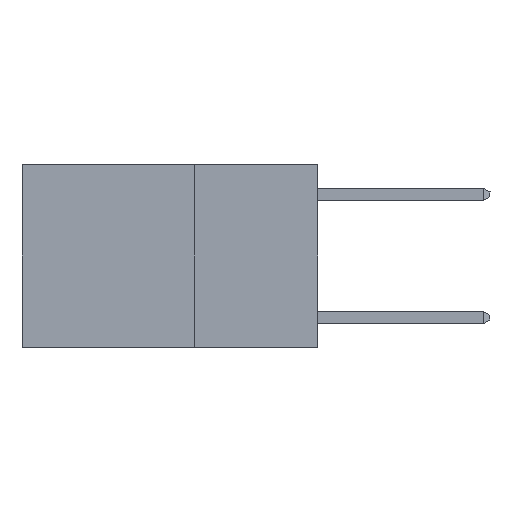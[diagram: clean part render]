
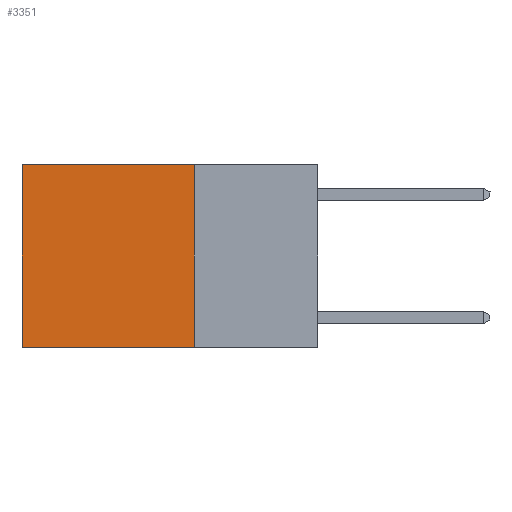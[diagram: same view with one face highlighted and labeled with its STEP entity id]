
A CAD part, left-side view. The second image highlights one B-rep face of the part: STEP entity #3351.
In plain terms, the highlighted planar face has unit normal (-1, 0, 0).
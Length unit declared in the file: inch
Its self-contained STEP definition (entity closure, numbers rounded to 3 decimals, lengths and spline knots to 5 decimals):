
#272 = VECTOR ( 'NONE', #531, 39.37008 ) ;
#531 = DIRECTION ( 'NONE',  ( 0., 0., -1. ) ) ;
#1153 = VERTEX_POINT ( 'NONE', #8296 ) ;
#1185 = CARTESIAN_POINT ( 'NONE',  ( 0.2625, 0.6, -0.37 ) ) ;
#1396 = LINE ( 'NONE', #9243, #9257 ) ;
#1548 = LINE ( 'NONE', #5243, #272 ) ;
#2403 = VERTEX_POINT ( 'NONE', #1185 ) ;
#2788 = VERTEX_POINT ( 'NONE', #6222 ) ;
#3244 = EDGE_LOOP ( 'NONE', ( #3820, #5809, #5583, #9516 ) ) ;
#3351 = ADVANCED_FACE ( 'NONE', ( #9793 ), #3911, .F. ) ;
#3608 = DIRECTION ( 'NONE',  ( 0., 0., -1. ) ) ;
#3707 = EDGE_CURVE ( 'NONE', #1153, #2403, #1548, .T. ) ;
#3820 = ORIENTED_EDGE ( 'NONE', *, *, #3707, .T. ) ;
#3834 = DIRECTION ( 'NONE',  ( 0., 0., -1. ) ) ;
#3839 = DIRECTION ( 'NONE',  ( 1., 0., 0. ) ) ;
#3861 = CARTESIAN_POINT ( 'NONE',  ( 0.2625, 0.25, 0. ) ) ;
#3911 = PLANE ( 'NONE',  #8380 ) ;
#4173 = DIRECTION ( 'NONE',  ( 0., 1., 0. ) ) ;
#4787 = LINE ( 'NONE', #7769, #7145 ) ;
#5030 = EDGE_CURVE ( 'NONE', #2788, #1153, #1396, .T. ) ;
#5243 = CARTESIAN_POINT ( 'NONE',  ( 0.2625, 0.6, 0. ) ) ;
#5583 = ORIENTED_EDGE ( 'NONE', *, *, #6615, .F. ) ;
#5777 = VECTOR ( 'NONE', #3608, 39.37008 ) ;
#5809 = ORIENTED_EDGE ( 'NONE', *, *, #5969, .F. ) ;
#5969 = EDGE_CURVE ( 'NONE', #9702, #2403, #4787, .T. ) ;
#6222 = CARTESIAN_POINT ( 'NONE',  ( 0.2625, 0.25, 0. ) ) ;
#6320 = DIRECTION ( 'NONE',  ( 0., 1., 0. ) ) ;
#6615 = EDGE_CURVE ( 'NONE', #2788, #9702, #9719, .T. ) ;
#7145 = VECTOR ( 'NONE', #4173, 39.37008 ) ;
#7769 = CARTESIAN_POINT ( 'NONE',  ( 0.2625, 0.25, -0.37 ) ) ;
#8296 = CARTESIAN_POINT ( 'NONE',  ( 0.2625, 0.6, 0. ) ) ;
#8380 = AXIS2_PLACEMENT_3D ( 'NONE', #3861, #3839, #3834 ) ;
#9243 = CARTESIAN_POINT ( 'NONE',  ( 0.2625, 0.25, 0. ) ) ;
#9257 = VECTOR ( 'NONE', #6320, 39.37008 ) ;
#9366 = CARTESIAN_POINT ( 'NONE',  ( 0.2625, 0.25, -0.37 ) ) ;
#9516 = ORIENTED_EDGE ( 'NONE', *, *, #5030, .T. ) ;
#9579 = CARTESIAN_POINT ( 'NONE',  ( 0.2625, 0.25, 0. ) ) ;
#9702 = VERTEX_POINT ( 'NONE', #9366 ) ;
#9719 = LINE ( 'NONE', #9579, #5777 ) ;
#9793 = FACE_OUTER_BOUND ( 'NONE', #3244, .T. ) ;
